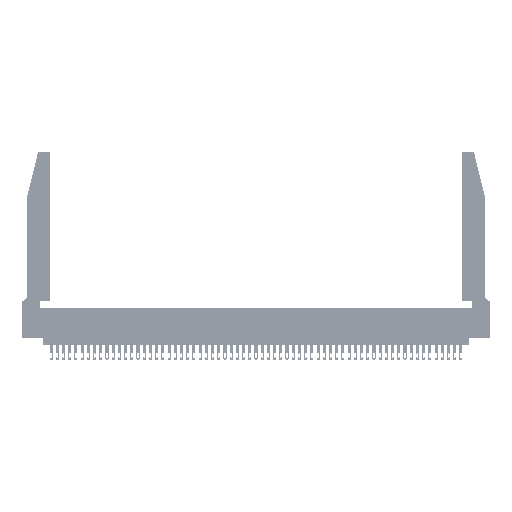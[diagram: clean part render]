
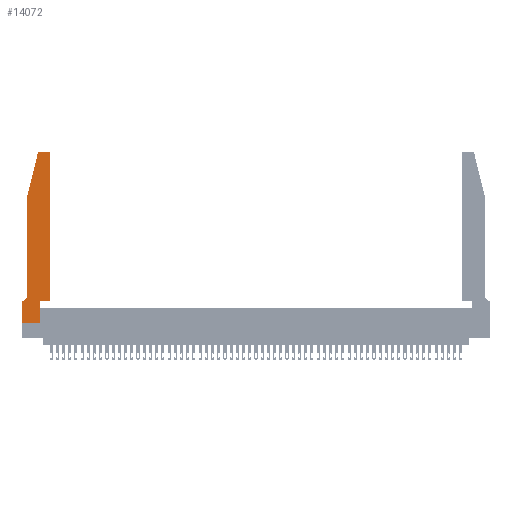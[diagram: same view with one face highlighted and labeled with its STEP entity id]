
A CAD part, top view. The second image highlights one B-rep face of the part: STEP entity #14072.
In plain terms, the highlighted planar face has unit normal (0, 0, 1).
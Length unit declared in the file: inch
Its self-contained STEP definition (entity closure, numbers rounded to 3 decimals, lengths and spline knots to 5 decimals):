
#447 = CARTESIAN_POINT ( 'NONE',  ( 0.4505, 0.35, 0.37 ) ) ;
#630 = VERTEX_POINT ( 'NONE', #8879 ) ;
#667 = CARTESIAN_POINT ( 'NONE',  ( 0.0755, 0.35, 0.37 ) ) ;
#2220 = CARTESIAN_POINT ( 'NONE',  ( 0.25487, 2.72718, 0.37 ) ) ;
#2617 = EDGE_CURVE ( 'NONE', #7531, #47115, #32099, .T. ) ;
#2634 = DIRECTION ( 'NONE',  ( 0., -1., 0. ) ) ;
#3993 = DIRECTION ( 'NONE',  ( 0., -1., 0. ) ) ;
#4150 = CARTESIAN_POINT ( 'NONE',  ( 0.0755, 2., 0.37 ) ) ;
#4483 = ORIENTED_EDGE ( 'NONE', *, *, #2617, .T. ) ;
#5218 = EDGE_CURVE ( 'NONE', #42902, #46316, #47442, .T. ) ;
#6538 = LINE ( 'NONE', #20583, #38474 ) ;
#7502 = CARTESIAN_POINT ( 'NONE',  ( 0.4205, 2.75, 0.37 ) ) ;
#7531 = VERTEX_POINT ( 'NONE', #44366 ) ;
#7553 = FACE_OUTER_BOUND ( 'NONE', #33216, .T. ) ;
#7747 = DIRECTION ( 'NONE',  ( 1., 0., 0. ) ) ;
#8726 = VECTOR ( 'NONE', #24950, 39.37008 ) ;
#8879 = CARTESIAN_POINT ( 'NONE',  ( 0.2865, 0., 0.37 ) ) ;
#9129 = CARTESIAN_POINT ( 'NONE',  ( 0.2605, 2.75, 0.37 ) ) ;
#9314 = ORIENTED_EDGE ( 'NONE', *, *, #13909, .T. ) ;
#10265 = ORIENTED_EDGE ( 'NONE', *, *, #15423, .T. ) ;
#11798 = CARTESIAN_POINT ( 'NONE',  ( 0.4505, 0.35, 0.37 ) ) ;
#12356 = LINE ( 'NONE', #667, #24128 ) ;
#12819 = DIRECTION ( 'NONE',  ( 0., 0., 1. ) ) ;
#13909 = EDGE_CURVE ( 'NONE', #16640, #47364, #16108, .T. ) ;
#14072 = ADVANCED_FACE ( 'NONE', ( #7553 ), #37242, .T. ) ;
#15423 = EDGE_CURVE ( 'NONE', #26758, #46147, #17260, .T. ) ;
#15621 = ORIENTED_EDGE ( 'NONE', *, *, #38365, .T. ) ;
#15953 = VECTOR ( 'NONE', #3993, 39.37008 ) ;
#16108 = LINE ( 'NONE', #40205, #44093 ) ;
#16193 = CARTESIAN_POINT ( 'NONE',  ( 0., 0., 0.37 ) ) ;
#16640 = VERTEX_POINT ( 'NONE', #36663 ) ;
#16876 = CARTESIAN_POINT ( 'NONE',  ( 0.284, 2.72, 0.37 ) ) ;
#17260 = CIRCLE ( 'NONE', #21979, 0.03 ) ;
#18429 = ORIENTED_EDGE ( 'NONE', *, *, #25588, .T. ) ;
#18553 = VECTOR ( 'NONE', #42982, 39.37008 ) ;
#19138 = VERTEX_POINT ( 'NONE', #40591 ) ;
#19490 = DIRECTION ( 'NONE',  ( 0., 1., 0. ) ) ;
#20227 = DIRECTION ( 'NONE',  ( 1., 0., 0. ) ) ;
#20530 = CARTESIAN_POINT ( 'NONE',  ( 0., 0.35, 0.37 ) ) ;
#20556 = CARTESIAN_POINT ( 'NONE',  ( 0.2865, 0.35, 0.37 ) ) ;
#20583 = CARTESIAN_POINT ( 'NONE',  ( 0.4505, 0.35, 0.37 ) ) ;
#20972 = DIRECTION ( 'NONE',  ( -1., 0., 0. ) ) ;
#21233 = DIRECTION ( 'NONE',  ( 1., 0., 0. ) ) ;
#21729 = VECTOR ( 'NONE', #7747, 39.37008 ) ;
#21979 = AXIS2_PLACEMENT_3D ( 'NONE', #16876, #54032, #21233 ) ;
#23326 = AXIS2_PLACEMENT_3D ( 'NONE', #20530, #12819, #25261 ) ;
#23451 = ORIENTED_EDGE ( 'NONE', *, *, #41529, .T. ) ;
#24128 = VECTOR ( 'NONE', #47559, 39.37008 ) ;
#24950 = DIRECTION ( 'NONE',  ( 1., 0., 0. ) ) ;
#25033 = CARTESIAN_POINT ( 'NONE',  ( 0.284, 2.75, 0.37 ) ) ;
#25261 = DIRECTION ( 'NONE',  ( 1., 0., 0. ) ) ;
#25588 = EDGE_CURVE ( 'NONE', #46147, #53487, #54020, .T. ) ;
#25715 = CARTESIAN_POINT ( 'NONE',  ( 0.0055, 0.35, 0.37 ) ) ;
#25941 = EDGE_CURVE ( 'NONE', #630, #19138, #29596, .T. ) ;
#25956 = EDGE_CURVE ( 'NONE', #47364, #630, #43241, .T. ) ;
#26123 = AXIS2_PLACEMENT_3D ( 'NONE', #29149, #33325, #20972 ) ;
#26421 = CARTESIAN_POINT ( 'NONE',  ( 0.0755, 2., 0.37 ) ) ;
#26758 = VERTEX_POINT ( 'NONE', #25033 ) ;
#27126 = CARTESIAN_POINT ( 'NONE',  ( 0., 0., 0.37 ) ) ;
#29149 = CARTESIAN_POINT ( 'NONE',  ( 0.0055, 0.42, 0.37 ) ) ;
#29596 = LINE ( 'NONE', #20556, #46547 ) ;
#29901 = ORIENTED_EDGE ( 'NONE', *, *, #5218, .T. ) ;
#29940 = ORIENTED_EDGE ( 'NONE', *, *, #25941, .T. ) ;
#30590 = ORIENTED_EDGE ( 'NONE', *, *, #25956, .T. ) ;
#32099 = CIRCLE ( 'NONE', #26123, 0.07 ) ;
#32588 = CARTESIAN_POINT ( 'NONE',  ( 0.4205, 2.72, 0.37 ) ) ;
#33216 = EDGE_LOOP ( 'NONE', ( #34748, #10265, #18429, #47672, #4483, #23451, #9314, #30590, #29940, #15621, #35184, #29901 ) ) ;
#33325 = DIRECTION ( 'NONE',  ( 0., 0., -1. ) ) ;
#33575 = LINE ( 'NONE', #9129, #47303 ) ;
#34309 = EDGE_CURVE ( 'NONE', #47640, #42902, #6538, .T. ) ;
#34748 = ORIENTED_EDGE ( 'NONE', *, *, #37479, .T. ) ;
#35184 = ORIENTED_EDGE ( 'NONE', *, *, #34309, .T. ) ;
#36110 = CARTESIAN_POINT ( 'NONE',  ( 0.4505, 2.72, 0.37 ) ) ;
#36663 = CARTESIAN_POINT ( 'NONE',  ( 0., 0.35, 0.37 ) ) ;
#37242 = PLANE ( 'NONE',  #23326 ) ;
#37479 = EDGE_CURVE ( 'NONE', #46316, #26758, #33575, .T. ) ;
#38365 = EDGE_CURVE ( 'NONE', #19138, #47640, #43321, .T. ) ;
#38474 = VECTOR ( 'NONE', #19490, 39.37008 ) ;
#40205 = CARTESIAN_POINT ( 'NONE',  ( 0., 0., 0.37 ) ) ;
#40591 = CARTESIAN_POINT ( 'NONE',  ( 0.2865, 0.35, 0.37 ) ) ;
#41391 = CARTESIAN_POINT ( 'NONE',  ( 0.0755, 2., 0.37 ) ) ;
#41529 = EDGE_CURVE ( 'NONE', #47115, #16640, #12356, .T. ) ;
#42902 = VERTEX_POINT ( 'NONE', #36110 ) ;
#42982 = DIRECTION ( 'NONE',  ( -0.239, -0.971, 0. ) ) ;
#43241 = LINE ( 'NONE', #16193, #21729 ) ;
#43321 = LINE ( 'NONE', #11798, #8726 ) ;
#43828 = DIRECTION ( 'NONE',  ( 0., 1., 0. ) ) ;
#44093 = VECTOR ( 'NONE', #2634, 39.37008 ) ;
#44366 = CARTESIAN_POINT ( 'NONE',  ( 0.0755, 0.42, 0.37 ) ) ;
#45011 = EDGE_CURVE ( 'NONE', #53487, #7531, #49178, .T. ) ;
#46147 = VERTEX_POINT ( 'NONE', #2220 ) ;
#46316 = VERTEX_POINT ( 'NONE', #7502 ) ;
#46547 = VECTOR ( 'NONE', #43828, 39.37008 ) ;
#47115 = VERTEX_POINT ( 'NONE', #25715 ) ;
#47303 = VECTOR ( 'NONE', #52315, 39.37008 ) ;
#47364 = VERTEX_POINT ( 'NONE', #27126 ) ;
#47442 = CIRCLE ( 'NONE', #52363, 0.03 ) ;
#47559 = DIRECTION ( 'NONE',  ( -1., 0., 0. ) ) ;
#47640 = VERTEX_POINT ( 'NONE', #447 ) ;
#47672 = ORIENTED_EDGE ( 'NONE', *, *, #45011, .T. ) ;
#48834 = DIRECTION ( 'NONE',  ( 0., 0., 1. ) ) ;
#49178 = LINE ( 'NONE', #41391, #15953 ) ;
#52315 = DIRECTION ( 'NONE',  ( -1., 0., 0. ) ) ;
#52363 = AXIS2_PLACEMENT_3D ( 'NONE', #32588, #48834, #20227 ) ;
#53487 = VERTEX_POINT ( 'NONE', #26421 ) ;
#54020 = LINE ( 'NONE', #4150, #18553 ) ;
#54032 = DIRECTION ( 'NONE',  ( 0., 0., 1. ) ) ;
